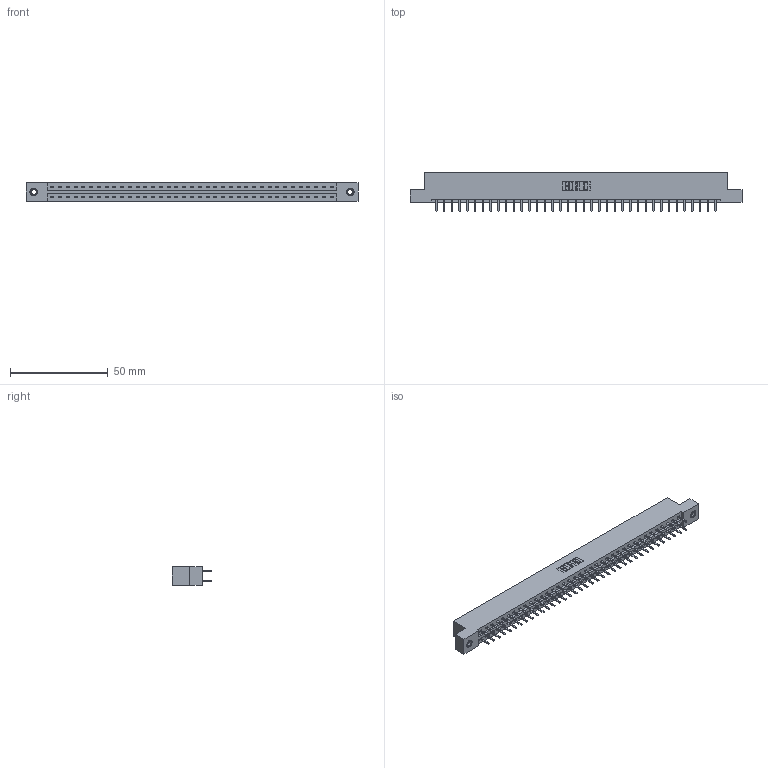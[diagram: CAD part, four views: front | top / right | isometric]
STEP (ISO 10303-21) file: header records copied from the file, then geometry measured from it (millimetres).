
FILE_DESCRIPTION (( 'STEP AP203' ), '1' );
FILE_NAME ('387-074-520-207.STEP', '2018-09-22T19:14:24', ( '' ), ( '' ), 'SwSTEP 2.0', 'SolidWorks 2016', '' );
FILE_SCHEMA (( 'CONFIG_CONTROL_DESIGN' ));
Length unit declared in the file: inch
Products named in the file (4): 337 Part_Flush Mounting Lugs - 0.156 Dia-TI; 345-292-001_345-293-120; 345-250-001_345-250-005-103; 387-074-520-207
Assembly tree (77 placements, depth 2):
  387-074-520-207
    337 Part_Flush Mounting Lugs - 0.156 Dia-TI
    345-292-001_345-293-120  x74
    345-250-001_345-250-005-103  x2
Bounding box: 169.62 x 20.02 x 9.4 mm (x, y, z)
Volume: 17763.4 mm3; surface area: 19976.2 mm2
Topology: 77 solids, 77 shells, 4466 faces, 12953 edges, 8430 vertices
Faces by surface type: plane 3062, cylinder 1388, cone 12, torus 4
Entity records: 30634 total; most frequent: CARTESIAN_POINT 5157, ORIENTED_EDGE 5074, DIRECTION 4415, EDGE_CURVE 2537, LINE 2385, VECTOR 2385, VERTEX_POINT 1684, AXIS2_PLACEMENT_3D 1015
